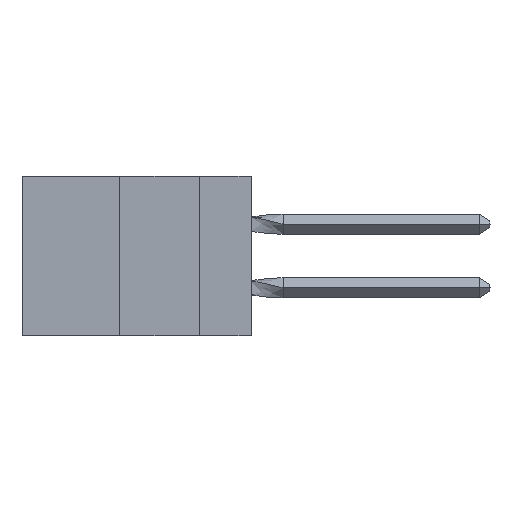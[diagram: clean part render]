
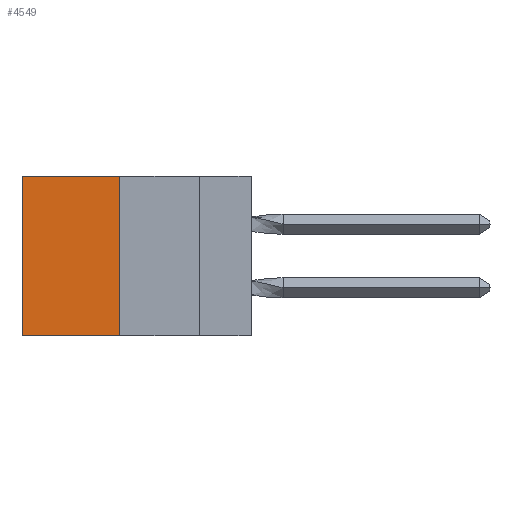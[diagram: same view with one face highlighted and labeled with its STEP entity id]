
A CAD part, left-side view. The second image highlights one B-rep face of the part: STEP entity #4549.
In plain terms, the highlighted planar face has unit normal (-1, 0, 0).
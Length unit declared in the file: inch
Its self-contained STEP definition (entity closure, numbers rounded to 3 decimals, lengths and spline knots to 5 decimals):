
#44 = CARTESIAN_POINT ( 'NONE',  ( 0.305, 0.413, -0.5 ) ) ;
#234 = CARTESIAN_POINT ( 'NONE',  ( 0.305, 0.413, -0.5 ) ) ;
#884 = FACE_OUTER_BOUND ( 'NONE', #7053, .T. ) ;
#1716 = DIRECTION ( 'NONE',  ( 0., 1., 0. ) ) ;
#3494 = LINE ( 'NONE', #12372, #19292 ) ;
#3679 = VECTOR ( 'NONE', #1716, 39.37008 ) ;
#3685 = DIRECTION ( 'NONE',  ( 0., 0., -1. ) ) ;
#3723 = VERTEX_POINT ( 'NONE', #234 ) ;
#3886 = DIRECTION ( 'NONE',  ( 1., 0., 0. ) ) ;
#3902 = ORIENTED_EDGE ( 'NONE', *, *, #16148, .T. ) ;
#4408 = ORIENTED_EDGE ( 'NONE', *, *, #15616, .F. ) ;
#4549 = ADVANCED_FACE ( 'NONE', ( #884 ), #6866, .F. ) ;
#5571 = CARTESIAN_POINT ( 'NONE',  ( 0.305, 0.413, -0.5 ) ) ;
#6179 = AXIS2_PLACEMENT_3D ( 'NONE', #13129, #3886, #3685 ) ;
#6866 = PLANE ( 'NONE',  #6179 ) ;
#7053 = EDGE_LOOP ( 'NONE', ( #19740, #16862, #4408, #3902 ) ) ;
#7361 = VERTEX_POINT ( 'NONE', #8575 ) ;
#7391 = LINE ( 'NONE', #44, #3679 ) ;
#8052 = CARTESIAN_POINT ( 'NONE',  ( 0.305, 0.72, 0. ) ) ;
#8575 = CARTESIAN_POINT ( 'NONE',  ( 0.305, 0.72, -0.5 ) ) ;
#8804 = EDGE_CURVE ( 'NONE', #3723, #7361, #7391, .T. ) ;
#9091 = CARTESIAN_POINT ( 'NONE',  ( 0.305, 0.413, 0. ) ) ;
#9284 = DIRECTION ( 'NONE',  ( 0., 0., -1. ) ) ;
#11366 = CARTESIAN_POINT ( 'NONE',  ( 0.305, 0.413, 0. ) ) ;
#11843 = VECTOR ( 'NONE', #19675, 39.37008 ) ;
#12372 = CARTESIAN_POINT ( 'NONE',  ( 0.305, 0.72, -0.5 ) ) ;
#13129 = CARTESIAN_POINT ( 'NONE',  ( 0.305, 0.413, -0.5 ) ) ;
#14499 = DIRECTION ( 'NONE',  ( 0., 1., 0. ) ) ;
#14732 = VECTOR ( 'NONE', #14499, 39.37008 ) ;
#15107 = VERTEX_POINT ( 'NONE', #9091 ) ;
#15616 = EDGE_CURVE ( 'NONE', #15107, #3723, #17463, .T. ) ;
#16020 = VERTEX_POINT ( 'NONE', #8052 ) ;
#16148 = EDGE_CURVE ( 'NONE', #15107, #16020, #19933, .T. ) ;
#16862 = ORIENTED_EDGE ( 'NONE', *, *, #8804, .F. ) ;
#17463 = LINE ( 'NONE', #5571, #11843 ) ;
#19292 = VECTOR ( 'NONE', #9284, 39.37008 ) ;
#19675 = DIRECTION ( 'NONE',  ( 0., 0., -1. ) ) ;
#19740 = ORIENTED_EDGE ( 'NONE', *, *, #20064, .T. ) ;
#19933 = LINE ( 'NONE', #11366, #14732 ) ;
#20064 = EDGE_CURVE ( 'NONE', #16020, #7361, #3494, .T. ) ;
